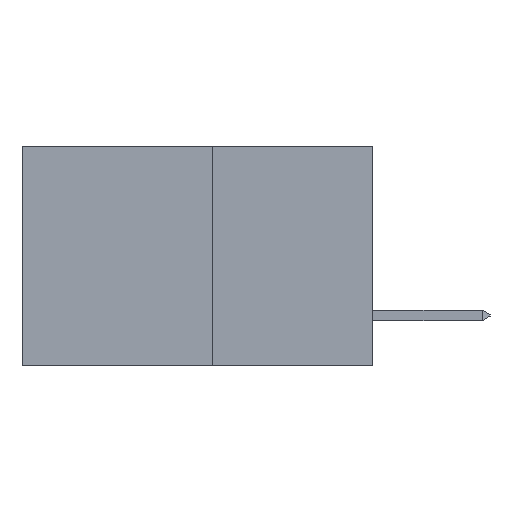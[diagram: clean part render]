
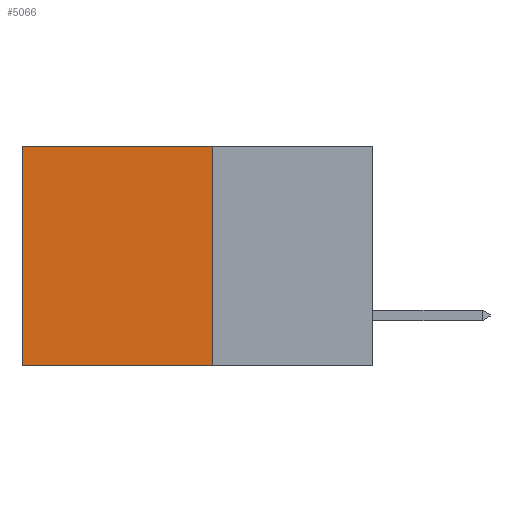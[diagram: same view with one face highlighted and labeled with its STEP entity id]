
A CAD part, left-side view. The second image highlights one B-rep face of the part: STEP entity #5066.
In plain terms, the highlighted planar face has unit normal (-1, 0, 0).
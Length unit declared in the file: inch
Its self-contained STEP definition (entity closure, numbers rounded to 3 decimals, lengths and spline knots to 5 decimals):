
#1 = LINE ( 'NONE', #1484, #6876 ) ;
#869 = CARTESIAN_POINT ( 'NONE',  ( 0.277, 0.59, 0. ) ) ;
#880 = CARTESIAN_POINT ( 'NONE',  ( 0.277, 0.27, 0. ) ) ;
#1484 = CARTESIAN_POINT ( 'NONE',  ( 0.277, 0.27, -0.37 ) ) ;
#1648 = ORIENTED_EDGE ( 'NONE', *, *, #10998, .F. ) ;
#2109 = EDGE_CURVE ( 'NONE', #5438, #3700, #7498, .T. ) ;
#2192 = ORIENTED_EDGE ( 'NONE', *, *, #5890, .F. ) ;
#2210 = CARTESIAN_POINT ( 'NONE',  ( 0.277, 0.27, -0.37 ) ) ;
#2754 = DIRECTION ( 'NONE',  ( 0., 0., -1. ) ) ;
#2781 = VECTOR ( 'NONE', #2754, 39.37008 ) ;
#3068 = ORIENTED_EDGE ( 'NONE', *, *, #2109, .T. ) ;
#3109 = DIRECTION ( 'NONE',  ( 0., 0., -1. ) ) ;
#3700 = VERTEX_POINT ( 'NONE', #6440 ) ;
#4386 = CARTESIAN_POINT ( 'NONE',  ( 0.277, 0.27, 0. ) ) ;
#4544 = FACE_OUTER_BOUND ( 'NONE', #7839, .T. ) ;
#4761 = ORIENTED_EDGE ( 'NONE', *, *, #9306, .T. ) ;
#4807 = CARTESIAN_POINT ( 'NONE',  ( 0.277, 0.27, -0.37 ) ) ;
#5066 = ADVANCED_FACE ( 'NONE', ( #4544 ), #9230, .F. ) ;
#5104 = DIRECTION ( 'NONE',  ( 0., 1., 0. ) ) ;
#5194 = CARTESIAN_POINT ( 'NONE',  ( 0.277, 0.27, -0.37 ) ) ;
#5366 = DIRECTION ( 'NONE',  ( 0., 1., 0. ) ) ;
#5438 = VERTEX_POINT ( 'NONE', #869 ) ;
#5890 = EDGE_CURVE ( 'NONE', #8851, #3700, #1, .T. ) ;
#6176 = LINE ( 'NONE', #880, #10244 ) ;
#6440 = CARTESIAN_POINT ( 'NONE',  ( 0.277, 0.59, -0.37 ) ) ;
#6566 = AXIS2_PLACEMENT_3D ( 'NONE', #2210, #8401, #3109 ) ;
#6646 = VERTEX_POINT ( 'NONE', #4386 ) ;
#6876 = VECTOR ( 'NONE', #5104, 39.37008 ) ;
#7498 = LINE ( 'NONE', #8234, #2781 ) ;
#7839 = EDGE_LOOP ( 'NONE', ( #3068, #2192, #1648, #4761 ) ) ;
#8234 = CARTESIAN_POINT ( 'NONE',  ( 0.277, 0.59, -0.37 ) ) ;
#8401 = DIRECTION ( 'NONE',  ( 1., 0., 0. ) ) ;
#8851 = VERTEX_POINT ( 'NONE', #4807 ) ;
#8985 = LINE ( 'NONE', #5194, #11025 ) ;
#9230 = PLANE ( 'NONE',  #6566 ) ;
#9306 = EDGE_CURVE ( 'NONE', #6646, #5438, #6176, .T. ) ;
#10244 = VECTOR ( 'NONE', #5366, 39.37008 ) ;
#10998 = EDGE_CURVE ( 'NONE', #6646, #8851, #8985, .T. ) ;
#11025 = VECTOR ( 'NONE', #11254, 39.37008 ) ;
#11254 = DIRECTION ( 'NONE',  ( 0., 0., -1. ) ) ;
